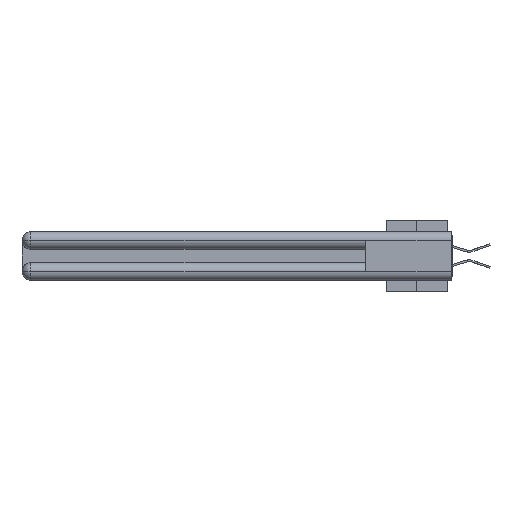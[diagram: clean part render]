
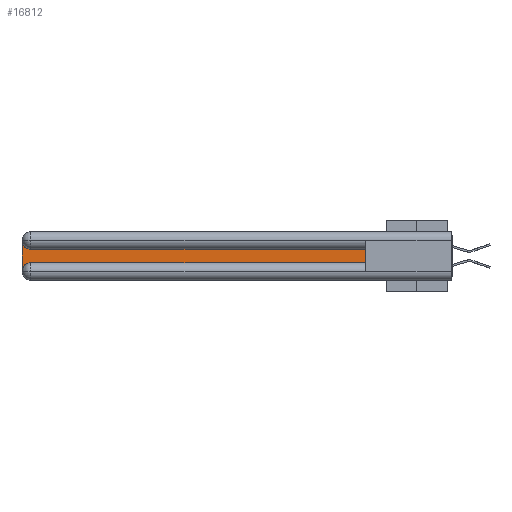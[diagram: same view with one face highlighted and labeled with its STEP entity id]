
A CAD part, left-side view. The second image highlights one B-rep face of the part: STEP entity #16812.
In plain terms, the highlighted planar face has unit normal (-1, 0, 0).
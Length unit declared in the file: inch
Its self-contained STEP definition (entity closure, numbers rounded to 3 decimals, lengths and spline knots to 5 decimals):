
#485 = VERTEX_POINT ( 'NONE', #2176 ) ;
#1407 = LINE ( 'NONE', #9726, #29206 ) ;
#1525 = VERTEX_POINT ( 'NONE', #13015 ) ;
#1573 = LINE ( 'NONE', #19357, #35286 ) ;
#2176 = CARTESIAN_POINT ( 'NONE',  ( 0.075, 0.6, -0.1225 ) ) ;
#2580 = CARTESIAN_POINT ( 'NONE',  ( 0.075, 0.6, -0.2175 ) ) ;
#3149 = VERTEX_POINT ( 'NONE', #4321 ) ;
#3692 = LINE ( 'NONE', #26551, #10420 ) ;
#4321 = CARTESIAN_POINT ( 'NONE',  ( 0.075, 2.94, -0.1225 ) ) ;
#5957 = EDGE_LOOP ( 'NONE', ( #9138, #9898, #22967, #11724, #18592, #31942 ) ) ;
#6171 = VERTEX_POINT ( 'NONE', #20625 ) ;
#8975 = EDGE_CURVE ( 'NONE', #6171, #16674, #21451, .T. ) ;
#9138 = ORIENTED_EDGE ( 'NONE', *, *, #28859, .T. ) ;
#9726 = CARTESIAN_POINT ( 'NONE',  ( 0.075, 3., -0.2175 ) ) ;
#9898 = ORIENTED_EDGE ( 'NONE', *, *, #32847, .T. ) ;
#10164 = CARTESIAN_POINT ( 'NONE',  ( 0.075, 2.94, -0.2775 ) ) ;
#10239 = DIRECTION ( 'NONE',  ( 0., 0., -1. ) ) ;
#10420 = VECTOR ( 'NONE', #15151, 39.37008 ) ;
#11621 = CIRCLE ( 'NONE', #19133, 0.06 ) ;
#11724 = ORIENTED_EDGE ( 'NONE', *, *, #8975, .T. ) ;
#12438 = DIRECTION ( 'NONE',  ( 0., 0., -1. ) ) ;
#12928 = CARTESIAN_POINT ( 'NONE',  ( 0.075, 3., -0.1225 ) ) ;
#13015 = CARTESIAN_POINT ( 'NONE',  ( 0.075, 3., -0.0625 ) ) ;
#13531 = DIRECTION ( 'NONE',  ( 1., 0., 0. ) ) ;
#13914 = DIRECTION ( 'NONE',  ( 0., 0., -1. ) ) ;
#15121 = VERTEX_POINT ( 'NONE', #21076 ) ;
#15151 = DIRECTION ( 'NONE',  ( 0., -1., 0. ) ) ;
#15674 = EDGE_CURVE ( 'NONE', #1525, #6171, #1407, .T. ) ;
#15706 = PLANE ( 'NONE',  #20000 ) ;
#15715 = DIRECTION ( 'NONE',  ( 0., 0., -1. ) ) ;
#16545 = CARTESIAN_POINT ( 'NONE',  ( 0.075, 2.94, -0.0625 ) ) ;
#16674 = VERTEX_POINT ( 'NONE', #32263 ) ;
#16812 = ADVANCED_FACE ( 'NONE', ( #21047 ), #15706, .F. ) ;
#16886 = DIRECTION ( 'NONE',  ( 0., 0., 1. ) ) ;
#18592 = ORIENTED_EDGE ( 'NONE', *, *, #31023, .T. ) ;
#18713 = DIRECTION ( 'NONE',  ( 1., 0., 0. ) ) ;
#19133 = AXIS2_PLACEMENT_3D ( 'NONE', #16545, #13531, #13914 ) ;
#19357 = CARTESIAN_POINT ( 'NONE',  ( 0.075, 0.6, -0.1225 ) ) ;
#19482 = LINE ( 'NONE', #2580, #23478 ) ;
#20000 = AXIS2_PLACEMENT_3D ( 'NONE', #12928, #23953, #12438 ) ;
#20318 = EDGE_CURVE ( 'NONE', #15121, #485, #19482, .T. ) ;
#20625 = CARTESIAN_POINT ( 'NONE',  ( 0.075, 3., -0.2775 ) ) ;
#21047 = FACE_OUTER_BOUND ( 'NONE', #5957, .T. ) ;
#21076 = CARTESIAN_POINT ( 'NONE',  ( 0.075, 0.6, -0.2175 ) ) ;
#21451 = CIRCLE ( 'NONE', #24598, 0.06 ) ;
#22224 = DIRECTION ( 'NONE',  ( 0., 1., 0. ) ) ;
#22967 = ORIENTED_EDGE ( 'NONE', *, *, #15674, .T. ) ;
#23478 = VECTOR ( 'NONE', #16886, 39.37008 ) ;
#23953 = DIRECTION ( 'NONE',  ( 1., 0., 0. ) ) ;
#24598 = AXIS2_PLACEMENT_3D ( 'NONE', #10164, #18713, #15715 ) ;
#26551 = CARTESIAN_POINT ( 'NONE',  ( 0.075, 0.6, -0.2175 ) ) ;
#28859 = EDGE_CURVE ( 'NONE', #485, #3149, #1573, .T. ) ;
#29206 = VECTOR ( 'NONE', #10239, 39.37008 ) ;
#31023 = EDGE_CURVE ( 'NONE', #16674, #15121, #3692, .T. ) ;
#31942 = ORIENTED_EDGE ( 'NONE', *, *, #20318, .T. ) ;
#32263 = CARTESIAN_POINT ( 'NONE',  ( 0.075, 2.94, -0.2175 ) ) ;
#32847 = EDGE_CURVE ( 'NONE', #3149, #1525, #11621, .T. ) ;
#35286 = VECTOR ( 'NONE', #22224, 39.37008 ) ;
